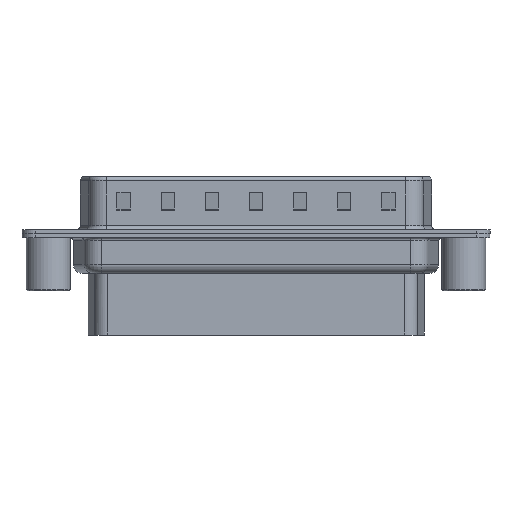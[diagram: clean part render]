
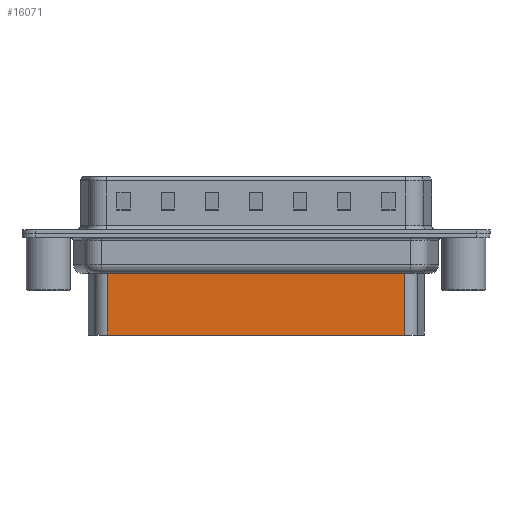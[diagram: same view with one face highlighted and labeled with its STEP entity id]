
A CAD part, front view. The second image highlights one B-rep face of the part: STEP entity #16071.
In plain terms, the highlighted planar face has unit normal (0, -1, 0).
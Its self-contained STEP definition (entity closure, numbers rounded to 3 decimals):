
#419 = DIRECTION ( 'NONE',  ( 0., 0., -1. ) ) ;
#484 = VERTEX_POINT ( 'NONE', #13740 ) ;
#693 = LINE ( 'NONE', #6983, #11783 ) ;
#1214 = ORIENTED_EDGE ( 'NONE', *, *, #1491, .F. ) ;
#1410 = LINE ( 'NONE', #11065, #16366 ) ;
#1491 = EDGE_CURVE ( 'NONE', #4123, #12043, #9530, .T. ) ;
#2408 = DIRECTION ( 'NONE',  ( -1., 0., 0. ) ) ;
#4123 = VERTEX_POINT ( 'NONE', #10686 ) ;
#4287 = LINE ( 'NONE', #9061, #11979 ) ;
#4808 = FACE_OUTER_BOUND ( 'NONE', #15450, .T. ) ;
#5592 = DIRECTION ( 'NONE',  ( -1., 0., 0. ) ) ;
#6117 = CARTESIAN_POINT ( 'NONE',  ( 40.344, -3.5, -3.1 ) ) ;
#6152 = VECTOR ( 'NONE', #17709, 1000. ) ;
#6564 = DIRECTION ( 'NONE',  ( 1., 0., 0. ) ) ;
#6983 = CARTESIAN_POINT ( 'NONE',  ( 6.706, -3.5, -11.45 ) ) ;
#9061 = CARTESIAN_POINT ( 'NONE',  ( 6.706, -3.5, -3.1 ) ) ;
#9512 = EDGE_CURVE ( 'NONE', #4123, #15698, #1410, .T. ) ;
#9530 = LINE ( 'NONE', #6117, #6152 ) ;
#9591 = ORIENTED_EDGE ( 'NONE', *, *, #10394, .T. ) ;
#10394 = EDGE_CURVE ( 'NONE', #15698, #484, #4287, .T. ) ;
#10686 = CARTESIAN_POINT ( 'NONE',  ( 40.344, -3.5, -4.097 ) ) ;
#10858 = CARTESIAN_POINT ( 'NONE',  ( 6.706, -3.5, -3.1 ) ) ;
#11065 = CARTESIAN_POINT ( 'NONE',  ( 6.459, -3.5, -4.097 ) ) ;
#11783 = VECTOR ( 'NONE', #5592, 1000. ) ;
#11979 = VECTOR ( 'NONE', #419, 1000. ) ;
#12043 = VERTEX_POINT ( 'NONE', #14098 ) ;
#13740 = CARTESIAN_POINT ( 'NONE',  ( 6.706, -3.5, -11.45 ) ) ;
#13809 = PLANE ( 'NONE',  #14366 ) ;
#14098 = CARTESIAN_POINT ( 'NONE',  ( 40.344, -3.5, -11.45 ) ) ;
#14366 = AXIS2_PLACEMENT_3D ( 'NONE', #10858, #15257, #6564 ) ;
#15257 = DIRECTION ( 'NONE',  ( 0., -1., 0. ) ) ;
#15450 = EDGE_LOOP ( 'NONE', ( #1214, #16957, #9591, #17985 ) ) ;
#15698 = VERTEX_POINT ( 'NONE', #16084 ) ;
#16071 = ADVANCED_FACE ( 'NONE', ( #4808 ), #13809, .T. ) ;
#16084 = CARTESIAN_POINT ( 'NONE',  ( 6.706, -3.5, -4.097 ) ) ;
#16366 = VECTOR ( 'NONE', #2408, 1000. ) ;
#16932 = EDGE_CURVE ( 'NONE', #12043, #484, #693, .T. ) ;
#16957 = ORIENTED_EDGE ( 'NONE', *, *, #9512, .T. ) ;
#17709 = DIRECTION ( 'NONE',  ( 0., 0., -1. ) ) ;
#17985 = ORIENTED_EDGE ( 'NONE', *, *, #16932, .F. ) ;
